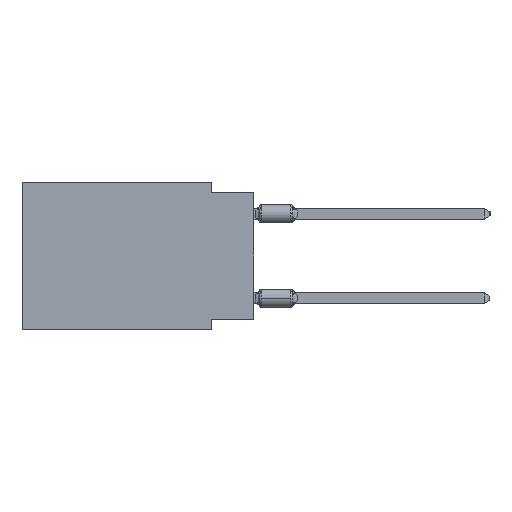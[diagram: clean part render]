
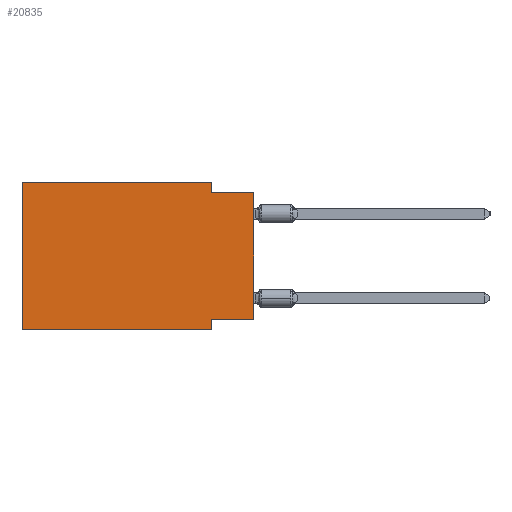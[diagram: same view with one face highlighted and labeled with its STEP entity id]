
A CAD part, left-side view. The second image highlights one B-rep face of the part: STEP entity #20835.
In plain terms, the highlighted planar face has unit normal (-1, 0, 0).
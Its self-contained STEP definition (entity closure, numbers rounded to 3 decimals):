
#1419 = EDGE_CURVE ( 'NONE', #46611, #41683, #7625, .T. ) ;
#2857 = CARTESIAN_POINT ( 'NONE',  ( 0., 13.97, -8.89 ) ) ;
#2992 = CARTESIAN_POINT ( 'NONE',  ( 0., 2.54, -8.89 ) ) ;
#4369 = LINE ( 'NONE', #44500, #13296 ) ;
#4924 = EDGE_CURVE ( 'NONE', #17918, #41683, #32893, .T. ) ;
#7625 = LINE ( 'NONE', #2857, #62243 ) ;
#9072 = CARTESIAN_POINT ( 'NONE',  ( 0., 0., -8.255 ) ) ;
#9572 = VECTOR ( 'NONE', #20025, 1000. ) ;
#10062 = VERTEX_POINT ( 'NONE', #9072 ) ;
#10884 = DIRECTION ( 'NONE',  ( 1., 0., 0. ) ) ;
#12254 = ORIENTED_EDGE ( 'NONE', *, *, #48210, .F. ) ;
#13296 = VECTOR ( 'NONE', #48644, 1000. ) ;
#13668 = EDGE_CURVE ( 'NONE', #18537, #58992, #26821, .T. ) ;
#14410 = EDGE_CURVE ( 'NONE', #10062, #17918, #28213, .T. ) ;
#14547 = EDGE_CURVE ( 'NONE', #48875, #41598, #39866, .T. ) ;
#15259 = CARTESIAN_POINT ( 'NONE',  ( 0., 2.54, -8.255 ) ) ;
#16209 = VECTOR ( 'NONE', #56346, 1000. ) ;
#16775 = ORIENTED_EDGE ( 'NONE', *, *, #4924, .F. ) ;
#17516 = LINE ( 'NONE', #36913, #16209 ) ;
#17822 = CARTESIAN_POINT ( 'NONE',  ( 0., 2.54, -8.89 ) ) ;
#17918 = VERTEX_POINT ( 'NONE', #15259 ) ;
#18537 = VERTEX_POINT ( 'NONE', #21342 ) ;
#19522 = CARTESIAN_POINT ( 'NONE',  ( 0., 0., -0.635 ) ) ;
#19803 = AXIS2_PLACEMENT_3D ( 'NONE', #35070, #10884, #59882 ) ;
#20025 = DIRECTION ( 'NONE',  ( 0., 0., 1. ) ) ;
#20835 = ADVANCED_FACE ( 'NONE', ( #44935 ), #40474, .F. ) ;
#21342 = CARTESIAN_POINT ( 'NONE',  ( 0., 13.97, 0. ) ) ;
#22069 = DIRECTION ( 'NONE',  ( 0., -1., 0. ) ) ;
#23656 = ORIENTED_EDGE ( 'NONE', *, *, #1419, .T. ) ;
#23979 = DIRECTION ( 'NONE',  ( 0., -1., 0. ) ) ;
#24640 = EDGE_CURVE ( 'NONE', #10062, #41598, #4369, .T. ) ;
#26109 = CARTESIAN_POINT ( 'NONE',  ( 0., 0., -0.635 ) ) ;
#26821 = LINE ( 'NONE', #59947, #40232 ) ;
#28213 = LINE ( 'NONE', #51773, #44321 ) ;
#28888 = VECTOR ( 'NONE', #51070, 1000. ) ;
#32893 = LINE ( 'NONE', #2992, #28888 ) ;
#33291 = DIRECTION ( 'NONE',  ( 0., 1., 0. ) ) ;
#33365 = ORIENTED_EDGE ( 'NONE', *, *, #41933, .F. ) ;
#34269 = ORIENTED_EDGE ( 'NONE', *, *, #14547, .F. ) ;
#35070 = CARTESIAN_POINT ( 'NONE',  ( 0., 13.97, 0. ) ) ;
#36226 = VECTOR ( 'NONE', #23979, 1000. ) ;
#36913 = CARTESIAN_POINT ( 'NONE',  ( 0., 2.54, 0. ) ) ;
#39191 = CARTESIAN_POINT ( 'NONE',  ( 0., 13.97, -8.89 ) ) ;
#39866 = LINE ( 'NONE', #19522, #36226 ) ;
#40232 = VECTOR ( 'NONE', #22069, 1000. ) ;
#40474 = PLANE ( 'NONE',  #19803 ) ;
#41598 = VERTEX_POINT ( 'NONE', #26109 ) ;
#41683 = VERTEX_POINT ( 'NONE', #17822 ) ;
#41933 = EDGE_CURVE ( 'NONE', #46611, #18537, #48672, .T. ) ;
#44210 = CARTESIAN_POINT ( 'NONE',  ( 0., 13.97, 0. ) ) ;
#44321 = VECTOR ( 'NONE', #33291, 1000. ) ;
#44500 = CARTESIAN_POINT ( 'NONE',  ( 0., 0., 0. ) ) ;
#44935 = FACE_OUTER_BOUND ( 'NONE', #49664, .T. ) ;
#46611 = VERTEX_POINT ( 'NONE', #39191 ) ;
#48210 = EDGE_CURVE ( 'NONE', #58992, #48875, #17516, .T. ) ;
#48535 = ORIENTED_EDGE ( 'NONE', *, *, #13668, .F. ) ;
#48644 = DIRECTION ( 'NONE',  ( 0., 0., 1. ) ) ;
#48672 = LINE ( 'NONE', #44210, #9572 ) ;
#48875 = VERTEX_POINT ( 'NONE', #60348 ) ;
#49664 = EDGE_LOOP ( 'NONE', ( #60791, #34269, #12254, #48535, #33365, #23656, #16775, #54650 ) ) ;
#51070 = DIRECTION ( 'NONE',  ( 0., 0., -1. ) ) ;
#51773 = CARTESIAN_POINT ( 'NONE',  ( 0., 0., -8.255 ) ) ;
#54650 = ORIENTED_EDGE ( 'NONE', *, *, #14410, .F. ) ;
#55399 = DIRECTION ( 'NONE',  ( 0., -1., 0. ) ) ;
#56346 = DIRECTION ( 'NONE',  ( 0., 0., -1. ) ) ;
#57645 = CARTESIAN_POINT ( 'NONE',  ( 0., 2.54, 0. ) ) ;
#58992 = VERTEX_POINT ( 'NONE', #57645 ) ;
#59882 = DIRECTION ( 'NONE',  ( 0., 0., -1. ) ) ;
#59947 = CARTESIAN_POINT ( 'NONE',  ( 0., 13.97, 0. ) ) ;
#60348 = CARTESIAN_POINT ( 'NONE',  ( 0., 2.54, -0.635 ) ) ;
#60791 = ORIENTED_EDGE ( 'NONE', *, *, #24640, .T. ) ;
#62243 = VECTOR ( 'NONE', #55399, 1000. ) ;
